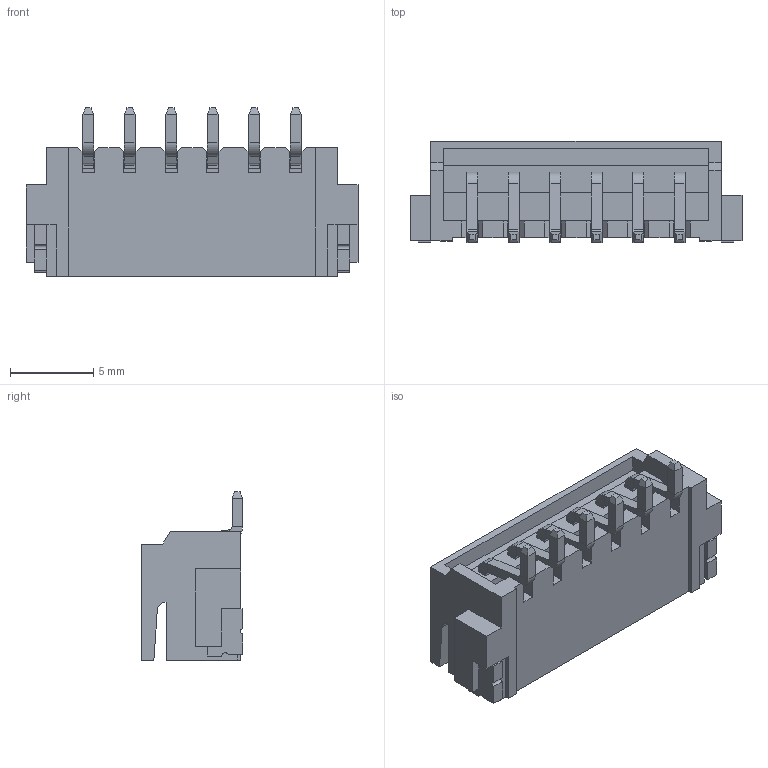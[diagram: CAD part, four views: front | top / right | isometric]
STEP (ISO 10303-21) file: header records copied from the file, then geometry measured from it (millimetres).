
FILE_DESCRIPTION (( 'STEP AP203' ), '1' );
FILE_NAME ('14K-506-418TAA1.STEP', '2024-02-22T13:20:29', ( '' ), ( '' ), 'SwSTEP 2.0', 'SolidWorks 2023', '' );
FILE_SCHEMA (( 'CONFIG_CONTROL_DESIGN' ));
Length unit declared in the file: millimetre
Products named in the file (3): 14K Series SMT Pin_Side Entry; 14K Series SMT Side Entry Insulator_506; 14K-506-418TAA1
Assembly tree (7 placements, depth 2):
  14K-506-418TAA1
    14K Series SMT Side Entry Insulator_506
    14K Series SMT Pin_Side Entry  x6
Bounding box: 20 x 6.1 x 10.15 mm (x, y, z)
Volume: 354.7 mm3; surface area: 1108.8 mm2
Topology: 7 solids, 7 shells, 397 faces, 985 edges, 602 vertices
Faces by surface type: plane 354, cylinder 43
Entity records: 7872 total; most frequent: CARTESIAN_POINT 1324, ORIENTED_EDGE 1310, DIRECTION 1195, EDGE_CURVE 655, LINE 609, VECTOR 609, VERTEX_POINT 422, AXIS2_PLACEMENT_3D 293
